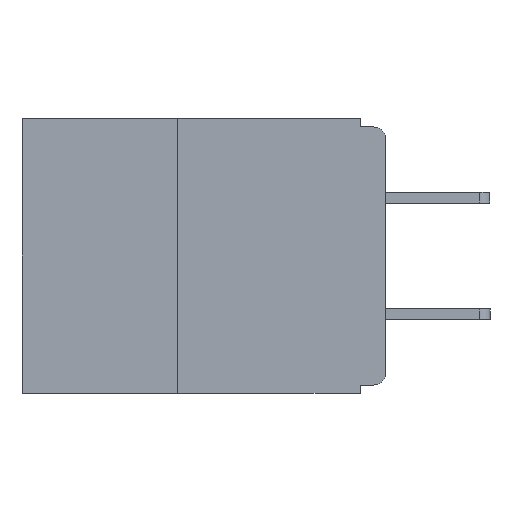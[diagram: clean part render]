
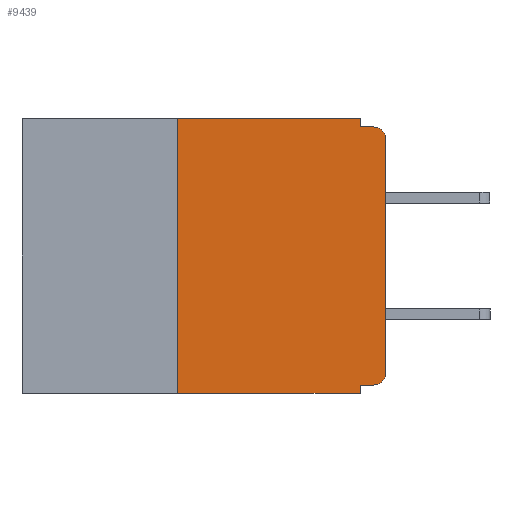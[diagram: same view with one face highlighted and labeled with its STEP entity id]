
A CAD part, left-side view. The second image highlights one B-rep face of the part: STEP entity #9439.
In plain terms, the highlighted planar face has unit normal (-1, 0, 0).
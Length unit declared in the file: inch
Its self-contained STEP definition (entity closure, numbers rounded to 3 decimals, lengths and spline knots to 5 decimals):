
#19 = DIRECTION ( 'NONE',  ( 0., -1., 0. ) ) ;
#259 = CARTESIAN_POINT ( 'NONE',  ( 0., 0.015, -0.01 ) ) ;
#452 = VECTOR ( 'NONE', #5603, 39.37008 ) ;
#500 = DIRECTION ( 'NONE',  ( 0., 0., -1. ) ) ;
#697 = EDGE_CURVE ( 'NONE', #11885, #1712, #11495, .T. ) ;
#736 = VECTOR ( 'NONE', #4425, 39.37008 ) ;
#865 = EDGE_CURVE ( 'NONE', #13639, #8771, #3238, .T. ) ;
#997 = CARTESIAN_POINT ( 'NONE',  ( 0., 0.25, -0.33 ) ) ;
#1712 = VERTEX_POINT ( 'NONE', #14593 ) ;
#2013 = EDGE_CURVE ( 'NONE', #1712, #6892, #6215, .T. ) ;
#2090 = VERTEX_POINT ( 'NONE', #5997 ) ;
#2178 = CIRCLE ( 'NONE', #11242, 0.015 ) ;
#2459 = VECTOR ( 'NONE', #500, 39.37008 ) ;
#2472 = EDGE_CURVE ( 'NONE', #2090, #6892, #7317, .T. ) ;
#2502 = CARTESIAN_POINT ( 'NONE',  ( 0., 0.437, 0. ) ) ;
#2541 = EDGE_LOOP ( 'NONE', ( #7922, #13074, #8309, #2636, #13102, #11498, #8737, #6264, #3440, #4947 ) ) ;
#2614 = CARTESIAN_POINT ( 'NONE',  ( 0., 0.015, -0.32 ) ) ;
#2636 = ORIENTED_EDGE ( 'NONE', *, *, #10573, .F. ) ;
#3061 = LINE ( 'NONE', #14333, #9131 ) ;
#3238 = LINE ( 'NONE', #4787, #15375 ) ;
#3440 = ORIENTED_EDGE ( 'NONE', *, *, #865, .F. ) ;
#3471 = DIRECTION ( 'NONE',  ( -1., 0., 0. ) ) ;
#4035 = LINE ( 'NONE', #12725, #736 ) ;
#4145 = AXIS2_PLACEMENT_3D ( 'NONE', #2502, #6169, #14377 ) ;
#4425 = DIRECTION ( 'NONE',  ( 0., 0., -1. ) ) ;
#4429 = DIRECTION ( 'NONE',  ( 0., 1., 0. ) ) ;
#4706 = DIRECTION ( 'NONE',  ( 0., 0., 1. ) ) ;
#4787 = CARTESIAN_POINT ( 'NONE',  ( 0., 0., -0.32 ) ) ;
#4890 = CARTESIAN_POINT ( 'NONE',  ( 0., 0., 0. ) ) ;
#4947 = ORIENTED_EDGE ( 'NONE', *, *, #15176, .T. ) ;
#5343 = CARTESIAN_POINT ( 'NONE',  ( 0., 0.437, -0.33 ) ) ;
#5603 = DIRECTION ( 'NONE',  ( 0., -1., 0. ) ) ;
#5692 = LINE ( 'NONE', #7803, #2459 ) ;
#5997 = CARTESIAN_POINT ( 'NONE',  ( 0., 0.031, -0.01 ) ) ;
#6169 = DIRECTION ( 'NONE',  ( 1., 0., 0. ) ) ;
#6215 = CIRCLE ( 'NONE', #14755, 0.015 ) ;
#6264 = ORIENTED_EDGE ( 'NONE', *, *, #13221, .F. ) ;
#6561 = DIRECTION ( 'NONE',  ( 0., -1., 0. ) ) ;
#6892 = VERTEX_POINT ( 'NONE', #259 ) ;
#7092 = CARTESIAN_POINT ( 'NONE',  ( 0., 0.25, 0. ) ) ;
#7317 = LINE ( 'NONE', #7520, #452 ) ;
#7330 = LINE ( 'NONE', #5343, #9804 ) ;
#7520 = CARTESIAN_POINT ( 'NONE',  ( 0., 0., -0.01 ) ) ;
#7649 = VERTEX_POINT ( 'NONE', #10196 ) ;
#7803 = CARTESIAN_POINT ( 'NONE',  ( 0., 0.031, -0.33 ) ) ;
#7922 = ORIENTED_EDGE ( 'NONE', *, *, #697, .T. ) ;
#7943 = LINE ( 'NONE', #997, #13439 ) ;
#8309 = ORIENTED_EDGE ( 'NONE', *, *, #2472, .F. ) ;
#8331 = VECTOR ( 'NONE', #10420, 39.37008 ) ;
#8737 = ORIENTED_EDGE ( 'NONE', *, *, #12540, .T. ) ;
#8771 = VERTEX_POINT ( 'NONE', #13215 ) ;
#8891 = DIRECTION ( 'NONE',  ( 0., 0., -1. ) ) ;
#8914 = DIRECTION ( 'NONE',  ( -1., 0., 0. ) ) ;
#8979 = CARTESIAN_POINT ( 'NONE',  ( 0., 0.015, -0.025 ) ) ;
#9131 = VECTOR ( 'NONE', #19, 39.37008 ) ;
#9439 = ADVANCED_FACE ( 'NONE', ( #13686 ), #10952, .F. ) ;
#9804 = VECTOR ( 'NONE', #6561, 39.37008 ) ;
#10196 = CARTESIAN_POINT ( 'NONE',  ( 0., 0.031, -0.33 ) ) ;
#10380 = CARTESIAN_POINT ( 'NONE',  ( 0., 0.031, 0. ) ) ;
#10420 = DIRECTION ( 'NONE',  ( 0., 0., 1. ) ) ;
#10554 = VERTEX_POINT ( 'NONE', #13831 ) ;
#10573 = EDGE_CURVE ( 'NONE', #13908, #2090, #4035, .T. ) ;
#10705 = CARTESIAN_POINT ( 'NONE',  ( 0., 0.015, -0.305 ) ) ;
#10952 = PLANE ( 'NONE',  #4145 ) ;
#11242 = AXIS2_PLACEMENT_3D ( 'NONE', #10705, #3471, #11838 ) ;
#11495 = LINE ( 'NONE', #4890, #8331 ) ;
#11498 = ORIENTED_EDGE ( 'NONE', *, *, #11859, .F. ) ;
#11838 = DIRECTION ( 'NONE',  ( 0., 0., -1. ) ) ;
#11859 = EDGE_CURVE ( 'NONE', #10554, #15362, #7943, .T. ) ;
#11885 = VERTEX_POINT ( 'NONE', #15251 ) ;
#12540 = EDGE_CURVE ( 'NONE', #10554, #7649, #7330, .T. ) ;
#12725 = CARTESIAN_POINT ( 'NONE',  ( 0., 0.031, 0. ) ) ;
#12948 = EDGE_CURVE ( 'NONE', #15362, #13908, #3061, .T. ) ;
#13074 = ORIENTED_EDGE ( 'NONE', *, *, #2013, .T. ) ;
#13102 = ORIENTED_EDGE ( 'NONE', *, *, #12948, .F. ) ;
#13215 = CARTESIAN_POINT ( 'NONE',  ( 0., 0.031, -0.32 ) ) ;
#13221 = EDGE_CURVE ( 'NONE', #8771, #7649, #5692, .T. ) ;
#13439 = VECTOR ( 'NONE', #4706, 39.37008 ) ;
#13639 = VERTEX_POINT ( 'NONE', #2614 ) ;
#13686 = FACE_OUTER_BOUND ( 'NONE', #2541, .T. ) ;
#13831 = CARTESIAN_POINT ( 'NONE',  ( 0., 0.25, -0.33 ) ) ;
#13908 = VERTEX_POINT ( 'NONE', #10380 ) ;
#14333 = CARTESIAN_POINT ( 'NONE',  ( 0., 0.437, 0. ) ) ;
#14377 = DIRECTION ( 'NONE',  ( 0., 0., -1. ) ) ;
#14593 = CARTESIAN_POINT ( 'NONE',  ( 0., 0., -0.025 ) ) ;
#14755 = AXIS2_PLACEMENT_3D ( 'NONE', #8979, #8914, #8891 ) ;
#15176 = EDGE_CURVE ( 'NONE', #13639, #11885, #2178, .T. ) ;
#15251 = CARTESIAN_POINT ( 'NONE',  ( 0., 0., -0.305 ) ) ;
#15362 = VERTEX_POINT ( 'NONE', #7092 ) ;
#15375 = VECTOR ( 'NONE', #4429, 39.37008 ) ;
